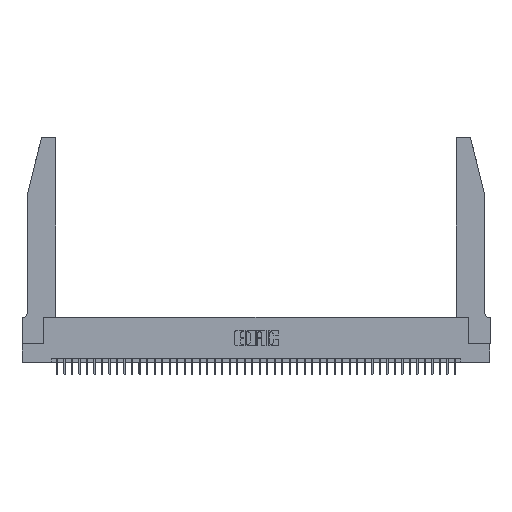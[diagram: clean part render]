
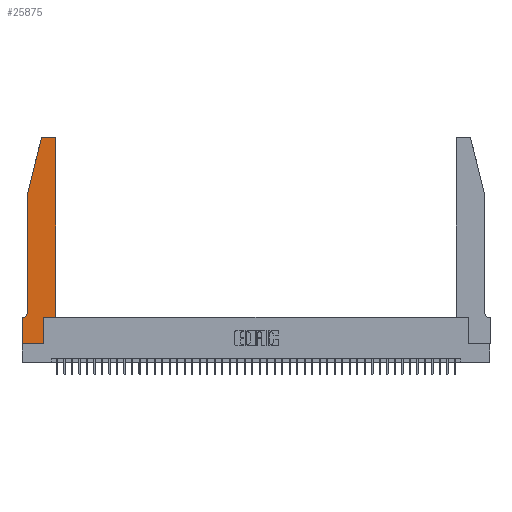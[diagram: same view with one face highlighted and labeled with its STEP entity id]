
A CAD part, top view. The second image highlights one B-rep face of the part: STEP entity #25875.
In plain terms, the highlighted planar face has unit normal (0, 0, 1).
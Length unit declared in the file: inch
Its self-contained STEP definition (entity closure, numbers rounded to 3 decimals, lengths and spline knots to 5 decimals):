
#231 = DIRECTION ( 'NONE',  ( 0., 0., 1. ) ) ;
#591 = CARTESIAN_POINT ( 'NONE',  ( 0.284, 2.72, 0.37 ) ) ;
#827 = LINE ( 'NONE', #15359, #27887 ) ;
#997 = CARTESIAN_POINT ( 'NONE',  ( 0.2605, 2.75, 0.37 ) ) ;
#1726 = LINE ( 'NONE', #997, #14415 ) ;
#1801 = CARTESIAN_POINT ( 'NONE',  ( 0.0055, 0.35, 0.37 ) ) ;
#1970 = CARTESIAN_POINT ( 'NONE',  ( 0., 0., 0.37 ) ) ;
#2167 = DIRECTION ( 'NONE',  ( 1., 0., 0. ) ) ;
#2954 = CARTESIAN_POINT ( 'NONE',  ( 0.284, 2.75, 0.37 ) ) ;
#3002 = EDGE_CURVE ( 'NONE', #19926, #12982, #44928, .T. ) ;
#3769 = EDGE_CURVE ( 'NONE', #32846, #44708, #28792, .T. ) ;
#5398 = DIRECTION ( 'NONE',  ( 0., 0., 1. ) ) ;
#5957 = CARTESIAN_POINT ( 'NONE',  ( 0.0755, 0.42, 0.37 ) ) ;
#5973 = ORIENTED_EDGE ( 'NONE', *, *, #3002, .T. ) ;
#6093 = CARTESIAN_POINT ( 'NONE',  ( 0.2865, 0., 0.37 ) ) ;
#6571 = ORIENTED_EDGE ( 'NONE', *, *, #7524, .T. ) ;
#6651 = DIRECTION ( 'NONE',  ( -1., 0., 0. ) ) ;
#7524 = EDGE_CURVE ( 'NONE', #23901, #21591, #20759, .T. ) ;
#7839 = DIRECTION ( 'NONE',  ( 1., 0., 0. ) ) ;
#8568 = EDGE_CURVE ( 'NONE', #12982, #23901, #41542, .T. ) ;
#9676 = EDGE_CURVE ( 'NONE', #44708, #19926, #40887, .T. ) ;
#9683 = VECTOR ( 'NONE', #12006, 39.37008 ) ;
#10570 = EDGE_CURVE ( 'NONE', #21591, #39701, #35532, .T. ) ;
#10829 = VECTOR ( 'NONE', #24725, 39.37008 ) ;
#11035 = VERTEX_POINT ( 'NONE', #30286 ) ;
#11489 = DIRECTION ( 'NONE',  ( 1., 0., 0. ) ) ;
#11516 = CARTESIAN_POINT ( 'NONE',  ( 0.0755, 2., 0.37 ) ) ;
#11909 = ORIENTED_EDGE ( 'NONE', *, *, #21885, .T. ) ;
#12006 = DIRECTION ( 'NONE',  ( -1., 0., 0. ) ) ;
#12031 = CARTESIAN_POINT ( 'NONE',  ( 0.4505, 0.35, 0.37 ) ) ;
#12254 = ORIENTED_EDGE ( 'NONE', *, *, #26449, .T. ) ;
#12971 = EDGE_LOOP ( 'NONE', ( #34483, #31715, #11909, #43811, #28928, #5973, #35540, #6571, #31662, #12254, #42125, #38175 ) ) ;
#12982 = VERTEX_POINT ( 'NONE', #14570 ) ;
#13187 = AXIS2_PLACEMENT_3D ( 'NONE', #591, #25307, #7839 ) ;
#13618 = DIRECTION ( 'NONE',  ( 0., 0., -1. ) ) ;
#14415 = VECTOR ( 'NONE', #29699, 39.37008 ) ;
#14427 = CARTESIAN_POINT ( 'NONE',  ( 0.0755, 2., 0.37 ) ) ;
#14570 = CARTESIAN_POINT ( 'NONE',  ( 0., 0.35, 0.37 ) ) ;
#15359 = CARTESIAN_POINT ( 'NONE',  ( 0.4505, 0.35, 0.37 ) ) ;
#15697 = VERTEX_POINT ( 'NONE', #12031 ) ;
#16086 = AXIS2_PLACEMENT_3D ( 'NONE', #35554, #231, #11489 ) ;
#17015 = CARTESIAN_POINT ( 'NONE',  ( 0.0055, 0.42, 0.37 ) ) ;
#17648 = EDGE_CURVE ( 'NONE', #24003, #11035, #22119, .T. ) ;
#18007 = LINE ( 'NONE', #24413, #10829 ) ;
#19926 = VERTEX_POINT ( 'NONE', #1801 ) ;
#20297 = CARTESIAN_POINT ( 'NONE',  ( 0.2865, 0.35, 0.37 ) ) ;
#20759 = LINE ( 'NONE', #24763, #24065 ) ;
#21059 = DIRECTION ( 'NONE',  ( 1., 0., 0. ) ) ;
#21591 = VERTEX_POINT ( 'NONE', #6093 ) ;
#21685 = CARTESIAN_POINT ( 'NONE',  ( 0.4505, 2.72, 0.37 ) ) ;
#21885 = EDGE_CURVE ( 'NONE', #24193, #32846, #28277, .T. ) ;
#22119 = CIRCLE ( 'NONE', #25099, 0.03 ) ;
#22141 = VECTOR ( 'NONE', #45468, 39.37008 ) ;
#23901 = VERTEX_POINT ( 'NONE', #28162 ) ;
#24003 = VERTEX_POINT ( 'NONE', #21685 ) ;
#24052 = EDGE_CURVE ( 'NONE', #15697, #24003, #827, .T. ) ;
#24065 = VECTOR ( 'NONE', #21059, 39.37008 ) ;
#24193 = VERTEX_POINT ( 'NONE', #44553 ) ;
#24323 = DIRECTION ( 'NONE',  ( -0.239, -0.971, 0. ) ) ;
#24413 = CARTESIAN_POINT ( 'NONE',  ( 0.4505, 0.35, 0.37 ) ) ;
#24725 = DIRECTION ( 'NONE',  ( 1., 0., 0. ) ) ;
#24763 = CARTESIAN_POINT ( 'NONE',  ( 0., 0., 0.37 ) ) ;
#24829 = CARTESIAN_POINT ( 'NONE',  ( 0.2865, 0.35, 0.37 ) ) ;
#25099 = AXIS2_PLACEMENT_3D ( 'NONE', #37012, #5398, #2167 ) ;
#25307 = DIRECTION ( 'NONE',  ( 0., 0., 1. ) ) ;
#25875 = ADVANCED_FACE ( 'NONE', ( #39203 ), #32478, .T. ) ;
#26005 = EDGE_CURVE ( 'NONE', #11035, #40947, #1726, .T. ) ;
#26449 = EDGE_CURVE ( 'NONE', #39701, #15697, #18007, .T. ) ;
#27046 = EDGE_CURVE ( 'NONE', #40947, #24193, #44733, .T. ) ;
#27887 = VECTOR ( 'NONE', #35694, 39.37008 ) ;
#28162 = CARTESIAN_POINT ( 'NONE',  ( 0., 0., 0.37 ) ) ;
#28277 = LINE ( 'NONE', #14427, #34336 ) ;
#28792 = LINE ( 'NONE', #35241, #22141 ) ;
#28922 = VECTOR ( 'NONE', #35452, 39.37008 ) ;
#28928 = ORIENTED_EDGE ( 'NONE', *, *, #9676, .T. ) ;
#29601 = DIRECTION ( 'NONE',  ( 0., -1., 0. ) ) ;
#29699 = DIRECTION ( 'NONE',  ( -1., 0., 0. ) ) ;
#30286 = CARTESIAN_POINT ( 'NONE',  ( 0.4205, 2.75, 0.37 ) ) ;
#31662 = ORIENTED_EDGE ( 'NONE', *, *, #10570, .T. ) ;
#31715 = ORIENTED_EDGE ( 'NONE', *, *, #27046, .T. ) ;
#32259 = VECTOR ( 'NONE', #29601, 39.37008 ) ;
#32478 = PLANE ( 'NONE',  #16086 ) ;
#32846 = VERTEX_POINT ( 'NONE', #11516 ) ;
#34336 = VECTOR ( 'NONE', #24323, 39.37008 ) ;
#34483 = ORIENTED_EDGE ( 'NONE', *, *, #26005, .T. ) ;
#35241 = CARTESIAN_POINT ( 'NONE',  ( 0.0755, 2., 0.37 ) ) ;
#35452 = DIRECTION ( 'NONE',  ( 0., 1., 0. ) ) ;
#35532 = LINE ( 'NONE', #24829, #28922 ) ;
#35540 = ORIENTED_EDGE ( 'NONE', *, *, #8568, .T. ) ;
#35554 = CARTESIAN_POINT ( 'NONE',  ( 0., 0.35, 0.37 ) ) ;
#35694 = DIRECTION ( 'NONE',  ( 0., 1., 0. ) ) ;
#37012 = CARTESIAN_POINT ( 'NONE',  ( 0.4205, 2.72, 0.37 ) ) ;
#37816 = AXIS2_PLACEMENT_3D ( 'NONE', #17015, #13618, #6651 ) ;
#38175 = ORIENTED_EDGE ( 'NONE', *, *, #17648, .T. ) ;
#39203 = FACE_OUTER_BOUND ( 'NONE', #12971, .T. ) ;
#39701 = VERTEX_POINT ( 'NONE', #20297 ) ;
#40887 = CIRCLE ( 'NONE', #37816, 0.07 ) ;
#40947 = VERTEX_POINT ( 'NONE', #2954 ) ;
#41542 = LINE ( 'NONE', #1970, #32259 ) ;
#42125 = ORIENTED_EDGE ( 'NONE', *, *, #24052, .T. ) ;
#43811 = ORIENTED_EDGE ( 'NONE', *, *, #3769, .T. ) ;
#44553 = CARTESIAN_POINT ( 'NONE',  ( 0.25487, 2.72718, 0.37 ) ) ;
#44625 = CARTESIAN_POINT ( 'NONE',  ( 0.0755, 0.35, 0.37 ) ) ;
#44708 = VERTEX_POINT ( 'NONE', #5957 ) ;
#44733 = CIRCLE ( 'NONE', #13187, 0.03 ) ;
#44928 = LINE ( 'NONE', #44625, #9683 ) ;
#45468 = DIRECTION ( 'NONE',  ( 0., -1., 0. ) ) ;
